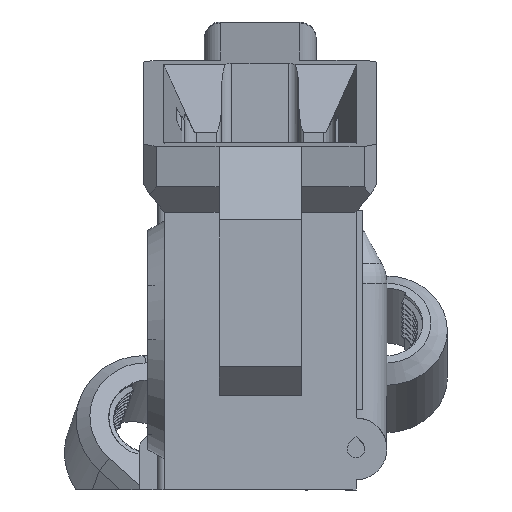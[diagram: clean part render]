
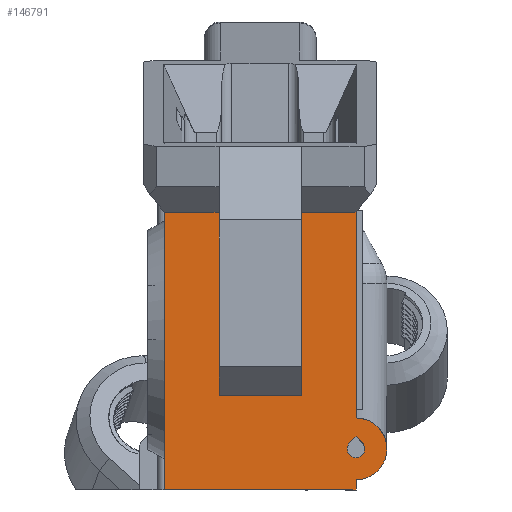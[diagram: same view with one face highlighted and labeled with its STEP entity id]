
A CAD part, left-side view. The second image highlights one B-rep face of the part: STEP entity #146791.
In plain terms, the highlighted planar face has unit normal (-1, 0, 0).
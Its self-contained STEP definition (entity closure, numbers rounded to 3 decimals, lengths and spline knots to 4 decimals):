
#3577 = EDGE_CURVE ( 'NONE', #175089, #75541, #150886, .T. ) ;
#5309 = DIRECTION ( 'NONE',  ( 0., 0.707, -0.707 ) ) ;
#6458 = CARTESIAN_POINT ( 'NONE',  ( -3.562, 0.6526, 2.518 ) ) ;
#10661 = CARTESIAN_POINT ( 'NONE',  ( -3.562, 0.3196, 0.8902 ) ) ;
#11293 = EDGE_CURVE ( 'NONE', #80155, #113563, #166736, .T. ) ;
#13303 = CARTESIAN_POINT ( 'NONE',  ( -3.562, 0.6526, 2.518 ) ) ;
#13415 = EDGE_CURVE ( 'NONE', #115887, #111676, #16121, .T. ) ;
#14777 = ORIENTED_EDGE ( 'NONE', *, *, #73572, .T. ) ;
#16121 = LINE ( 'NONE', #39800, #168493 ) ;
#17669 = EDGE_CURVE ( 'NONE', #79071, #66691, #48192, .T. ) ;
#17857 = VECTOR ( 'NONE', #5309, 39.3701 ) ;
#18936 = DIRECTION ( 'NONE',  ( -1., 0., 0. ) ) ;
#24093 = VECTOR ( 'NONE', #90013, 39.3701 ) ;
#27218 = VECTOR ( 'NONE', #61089, 39.3701 ) ;
#27964 = ORIENTED_EDGE ( 'NONE', *, *, #151744, .T. ) ;
#30291 = CARTESIAN_POINT ( 'NONE',  ( -3.562, 0.3196, 1.1538 ) ) ;
#31149 = DIRECTION ( 'NONE',  ( 0., 0., -1. ) ) ;
#31594 = LINE ( 'NONE', #47077, #27218 ) ;
#39800 = CARTESIAN_POINT ( 'NONE',  ( -3.562, 0.3196, 1.8282 ) ) ;
#44849 = ORIENTED_EDGE ( 'NONE', *, *, #157178, .F. ) ;
#45947 = LINE ( 'NONE', #162057, #52606 ) ;
#45987 = LINE ( 'NONE', #101170, #148273 ) ;
#47077 = CARTESIAN_POINT ( 'NONE',  ( -3.562, -0.1474, 2.518 ) ) ;
#48192 = CIRCLE ( 'NONE', #132013, 0.0534 ) ;
#48230 = CIRCLE ( 'NONE', #170215, 0.0534 ) ;
#49230 = CIRCLE ( 'NONE', #110941, 0.188 ) ;
#49675 = PLANE ( 'NONE',  #75179 ) ;
#50297 = VECTOR ( 'NONE', #149579, 39.3701 ) ;
#52606 = VECTOR ( 'NONE', #117756, 39.3701 ) ;
#53322 = CARTESIAN_POINT ( 'NONE',  ( -3.562, 1.4856, 0.8282 ) ) ;
#53605 = EDGE_LOOP ( 'NONE', ( #125284, #14777, #98430, #56790, #58608, #57427, #179926, #166989, #110626, #27964 ) ) ;
#55035 = DIRECTION ( 'NONE',  ( 0., 0., -1. ) ) ;
#56790 = ORIENTED_EDGE ( 'NONE', *, *, #99809, .T. ) ;
#57363 = VECTOR ( 'NONE', #156621, 39.3701 ) ;
#57427 = ORIENTED_EDGE ( 'NONE', *, *, #3577, .T. ) ;
#58608 = ORIENTED_EDGE ( 'NONE', *, *, #139513, .F. ) ;
#61089 = DIRECTION ( 'NONE',  ( 0., 1., 0. ) ) ;
#61796 = EDGE_CURVE ( 'NONE', #75541, #113563, #127635, .T. ) ;
#62941 = FACE_OUTER_BOUND ( 'NONE', #53605, .T. ) ;
#63678 = CARTESIAN_POINT ( 'NONE',  ( -3.562, 0.3196, 0.8282 ) ) ;
#66613 = VERTEX_POINT ( 'NONE', #138764 ) ;
#66691 = VERTEX_POINT ( 'NONE', #84559 ) ;
#71994 = DIRECTION ( 'NONE',  ( 0., 0., -1. ) ) ;
#73572 = EDGE_CURVE ( 'NONE', #107917, #111676, #169972, .T. ) ;
#75179 = AXIS2_PLACEMENT_3D ( 'NONE', #76449, #161510, #91591 ) ;
#75541 = VERTEX_POINT ( 'NONE', #6458 ) ;
#76449 = CARTESIAN_POINT ( 'NONE',  ( -3.562, 0.6526, 1.8282 ) ) ;
#77021 = VERTEX_POINT ( 'NONE', #89861 ) ;
#77725 = VERTEX_POINT ( 'NONE', #95610 ) ;
#79071 = VERTEX_POINT ( 'NONE', #85084 ) ;
#80155 = VERTEX_POINT ( 'NONE', #119780 ) ;
#81886 = VECTOR ( 'NONE', #143428, 39.3701 ) ;
#84559 = CARTESIAN_POINT ( 'NONE',  ( -3.562, 0.2818, 1.116 ) ) ;
#85084 = CARTESIAN_POINT ( 'NONE',  ( -3.562, 0.3196, 1.0248 ) ) ;
#87418 = DIRECTION ( 'NONE',  ( 0., 0., 1. ) ) ;
#89861 = CARTESIAN_POINT ( 'NONE',  ( -3.562, 0.3196, 1.2662 ) ) ;
#90013 = DIRECTION ( 'NONE',  ( 0., 0.707, 0.707 ) ) ;
#91591 = DIRECTION ( 'NONE',  ( 0., 0., 1. ) ) ;
#93439 = CARTESIAN_POINT ( 'NONE',  ( -3.562, 0.6526, 1.4032 ) ) ;
#94682 = ORIENTED_EDGE ( 'NONE', *, *, #17669, .F. ) ;
#95610 = CARTESIAN_POINT ( 'NONE',  ( -3.562, 0.3574, 1.116 ) ) ;
#98430 = ORIENTED_EDGE ( 'NONE', *, *, #13415, .F. ) ;
#99809 = EDGE_CURVE ( 'NONE', #115887, #77021, #49230, .T. ) ;
#100474 = CARTESIAN_POINT ( 'NONE',  ( -3.562, 0.3196, 1.0782 ) ) ;
#101170 = CARTESIAN_POINT ( 'NONE',  ( -3.562, 1.4856, 1.8282 ) ) ;
#101697 = ORIENTED_EDGE ( 'NONE', *, *, #173916, .F. ) ;
#105734 = CARTESIAN_POINT ( 'NONE',  ( -3.562, 0.3196, 1.1538 ) ) ;
#107556 = VECTOR ( 'NONE', #137121, 39.3701 ) ;
#107917 = VERTEX_POINT ( 'NONE', #53322 ) ;
#109684 = DIRECTION ( 'NONE',  ( -1., 0., 0. ) ) ;
#110626 = ORIENTED_EDGE ( 'NONE', *, *, #142737, .F. ) ;
#110941 = AXIS2_PLACEMENT_3D ( 'NONE', #154962, #170692, #87418 ) ;
#111676 = VERTEX_POINT ( 'NONE', #63678 ) ;
#113563 = VERTEX_POINT ( 'NONE', #93439 ) ;
#115887 = VERTEX_POINT ( 'NONE', #10661 ) ;
#117756 = DIRECTION ( 'NONE',  ( 0., 0., -1. ) ) ;
#117769 = ORIENTED_EDGE ( 'NONE', *, *, #166188, .F. ) ;
#118320 = EDGE_LOOP ( 'NONE', ( #44849, #117769, #101697, #94682 ) ) ;
#119780 = CARTESIAN_POINT ( 'NONE',  ( -3.562, 1.1526, 1.4032 ) ) ;
#122464 = DIRECTION ( 'NONE',  ( 0., 0., -1. ) ) ;
#123995 = CARTESIAN_POINT ( 'NONE',  ( -3.562, 2.4558, 1.4032 ) ) ;
#125284 = ORIENTED_EDGE ( 'NONE', *, *, #168407, .T. ) ;
#127635 = LINE ( 'NONE', #13303, #81886 ) ;
#132013 = AXIS2_PLACEMENT_3D ( 'NONE', #178373, #109684, #122464 ) ;
#137121 = DIRECTION ( 'NONE',  ( 0., 0., -1. ) ) ;
#138764 = CARTESIAN_POINT ( 'NONE',  ( -3.562, 1.4856, 2.518 ) ) ;
#139174 = DIRECTION ( 'NONE',  ( 0., -1., 0. ) ) ;
#139513 = EDGE_CURVE ( 'NONE', #175089, #77021, #157633, .T. ) ;
#142737 = EDGE_CURVE ( 'NONE', #150400, #80155, #45947, .T. ) ;
#143428 = DIRECTION ( 'NONE',  ( 0., 0., -1. ) ) ;
#146791 = ADVANCED_FACE ( 'NONE', ( #62941, #152109 ), #49675, .F. ) ;
#148273 = VECTOR ( 'NONE', #71994, 39.3701 ) ;
#149579 = DIRECTION ( 'NONE',  ( 0., -1., 0. ) ) ;
#150400 = VERTEX_POINT ( 'NONE', #168604 ) ;
#150755 = CARTESIAN_POINT ( 'NONE',  ( -3.562, 0.3196, 2.518 ) ) ;
#150886 = LINE ( 'NONE', #157217, #57363 ) ;
#151744 = EDGE_CURVE ( 'NONE', #150400, #66613, #31594, .T. ) ;
#152109 = FACE_BOUND ( 'NONE', #118320, .T. ) ;
#154962 = CARTESIAN_POINT ( 'NONE',  ( -3.562, 0.3196, 1.0782 ) ) ;
#156621 = DIRECTION ( 'NONE',  ( 0., 1., 0. ) ) ;
#157178 = EDGE_CURVE ( 'NONE', #77725, #79071, #48230, .T. ) ;
#157217 = CARTESIAN_POINT ( 'NONE',  ( -3.562, -0.1474, 2.518 ) ) ;
#157633 = LINE ( 'NONE', #166796, #107556 ) ;
#158743 = CARTESIAN_POINT ( 'NONE',  ( -3.562, 0.2818, 1.116 ) ) ;
#159000 = LINE ( 'NONE', #158743, #24093 ) ;
#161510 = DIRECTION ( 'NONE',  ( 1., 0., 0. ) ) ;
#162057 = CARTESIAN_POINT ( 'NONE',  ( -3.562, 1.1526, 0.8282 ) ) ;
#162381 = VECTOR ( 'NONE', #139174, 39.3701 ) ;
#165351 = CARTESIAN_POINT ( 'NONE',  ( -3.562, 0.6526, 0.8282 ) ) ;
#166188 = EDGE_CURVE ( 'NONE', #175472, #77725, #172467, .T. ) ;
#166736 = LINE ( 'NONE', #123995, #162381 ) ;
#166796 = CARTESIAN_POINT ( 'NONE',  ( -3.562, 0.3196, 3.2514 ) ) ;
#166989 = ORIENTED_EDGE ( 'NONE', *, *, #11293, .F. ) ;
#168407 = EDGE_CURVE ( 'NONE', #66613, #107917, #45987, .T. ) ;
#168493 = VECTOR ( 'NONE', #55035, 39.3701 ) ;
#168604 = CARTESIAN_POINT ( 'NONE',  ( -3.562, 1.1526, 2.518 ) ) ;
#169972 = LINE ( 'NONE', #165351, #50297 ) ;
#170215 = AXIS2_PLACEMENT_3D ( 'NONE', #100474, #18936, #31149 ) ;
#170692 = DIRECTION ( 'NONE',  ( -1., 0., 0. ) ) ;
#172467 = LINE ( 'NONE', #105734, #17857 ) ;
#173916 = EDGE_CURVE ( 'NONE', #66691, #175472, #159000, .T. ) ;
#175089 = VERTEX_POINT ( 'NONE', #150755 ) ;
#175472 = VERTEX_POINT ( 'NONE', #30291 ) ;
#178373 = CARTESIAN_POINT ( 'NONE',  ( -3.562, 0.3196, 1.0782 ) ) ;
#179926 = ORIENTED_EDGE ( 'NONE', *, *, #61796, .T. ) ;
